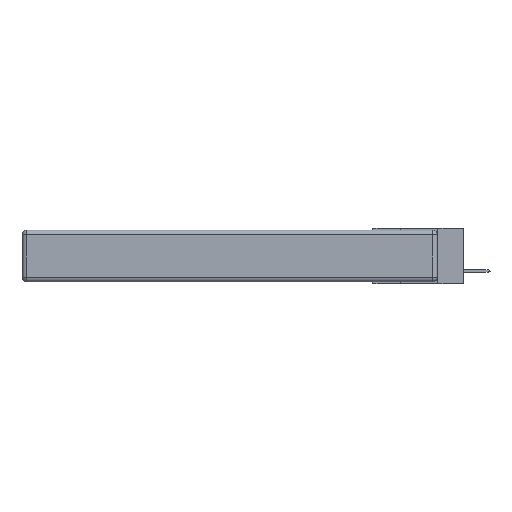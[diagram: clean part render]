
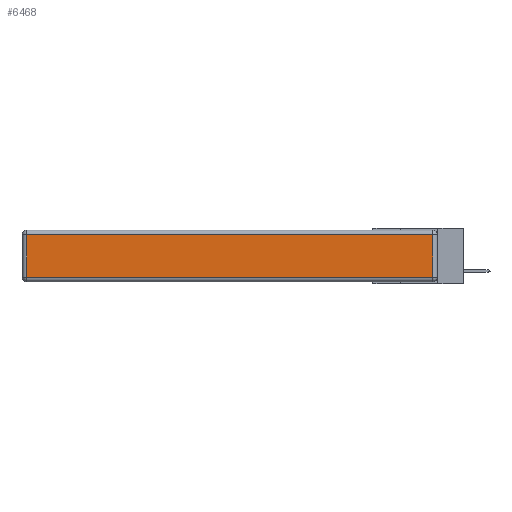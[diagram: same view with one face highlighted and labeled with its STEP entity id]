
A CAD part, left-side view. The second image highlights one B-rep face of the part: STEP entity #6468.
In plain terms, the highlighted planar face has unit normal (-1, 0, 0).
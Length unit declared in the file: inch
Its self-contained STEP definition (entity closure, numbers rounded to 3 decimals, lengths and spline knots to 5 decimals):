
#118 = PLANE ( 'NONE',  #9486 ) ;
#193 = LINE ( 'NONE', #1386, #11010 ) ;
#377 = VECTOR ( 'NONE', #5698, 39.37008 ) ;
#486 = DIRECTION ( 'NONE',  ( 0., -1., 0. ) ) ;
#574 = EDGE_CURVE ( 'NONE', #5197, #1799, #193, .T. ) ;
#750 = CARTESIAN_POINT ( 'NONE',  ( 0., 2.72, -0.343 ) ) ;
#1386 = CARTESIAN_POINT ( 'NONE',  ( 0., 0.03, -0.343 ) ) ;
#1799 = VERTEX_POINT ( 'NONE', #2381 ) ;
#2381 = CARTESIAN_POINT ( 'NONE',  ( 0., 0.03, -0.03 ) ) ;
#2625 = CARTESIAN_POINT ( 'NONE',  ( 0., 2.72, -0.313 ) ) ;
#2648 = ORIENTED_EDGE ( 'NONE', *, *, #574, .T. ) ;
#2901 = CARTESIAN_POINT ( 'NONE',  ( 0., 2.75, -0.03 ) ) ;
#3114 = EDGE_CURVE ( 'NONE', #4826, #10641, #3468, .T. ) ;
#3468 = LINE ( 'NONE', #750, #11954 ) ;
#3948 = DIRECTION ( 'NONE',  ( 0., 0., 1. ) ) ;
#4826 = VERTEX_POINT ( 'NONE', #11027 ) ;
#4842 = VECTOR ( 'NONE', #486, 39.37008 ) ;
#4849 = CARTESIAN_POINT ( 'NONE',  ( 0., 0., -0.343 ) ) ;
#4882 = ORIENTED_EDGE ( 'NONE', *, *, #3114, .T. ) ;
#5197 = VERTEX_POINT ( 'NONE', #6985 ) ;
#5698 = DIRECTION ( 'NONE',  ( 0., 1., 0. ) ) ;
#6468 = ADVANCED_FACE ( 'NONE', ( #6625 ), #118, .T. ) ;
#6625 = FACE_OUTER_BOUND ( 'NONE', #9312, .T. ) ;
#6705 = DIRECTION ( 'NONE',  ( -1., 0., 0. ) ) ;
#6882 = EDGE_CURVE ( 'NONE', #10641, #5197, #9838, .T. ) ;
#6985 = CARTESIAN_POINT ( 'NONE',  ( 0., 0.03, -0.313 ) ) ;
#8904 = CARTESIAN_POINT ( 'NONE',  ( 0., 0., -0.313 ) ) ;
#9058 = ORIENTED_EDGE ( 'NONE', *, *, #6882, .T. ) ;
#9168 = DIRECTION ( 'NONE',  ( 0., 0., -1. ) ) ;
#9312 = EDGE_LOOP ( 'NONE', ( #9058, #2648, #12090, #4882 ) ) ;
#9486 = AXIS2_PLACEMENT_3D ( 'NONE', #4849, #6705, #3948 ) ;
#9838 = LINE ( 'NONE', #8904, #4842 ) ;
#10308 = LINE ( 'NONE', #2901, #377 ) ;
#10396 = EDGE_CURVE ( 'NONE', #1799, #4826, #10308, .T. ) ;
#10641 = VERTEX_POINT ( 'NONE', #2625 ) ;
#11010 = VECTOR ( 'NONE', #11794, 39.37008 ) ;
#11027 = CARTESIAN_POINT ( 'NONE',  ( 0., 2.72, -0.03 ) ) ;
#11794 = DIRECTION ( 'NONE',  ( 0., 0., 1. ) ) ;
#11954 = VECTOR ( 'NONE', #9168, 39.37008 ) ;
#12090 = ORIENTED_EDGE ( 'NONE', *, *, #10396, .T. ) ;
